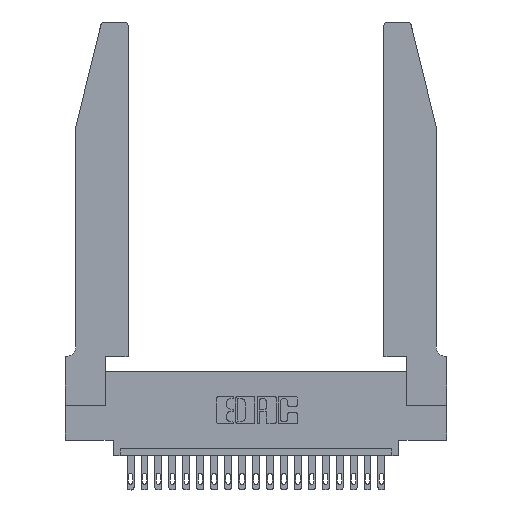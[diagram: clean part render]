
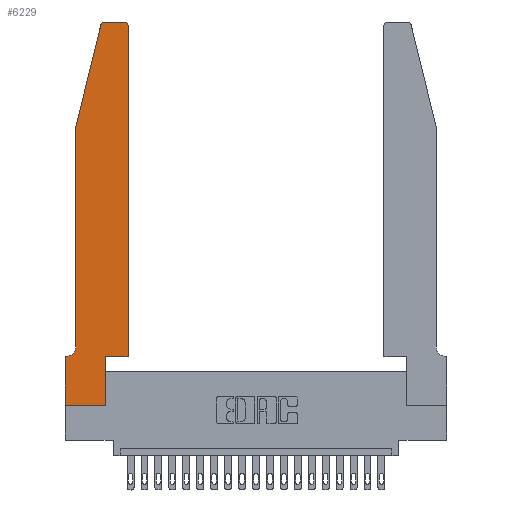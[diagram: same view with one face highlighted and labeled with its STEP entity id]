
A CAD part, top view. The second image highlights one B-rep face of the part: STEP entity #6229.
In plain terms, the highlighted planar face has unit normal (0, 0, 1).
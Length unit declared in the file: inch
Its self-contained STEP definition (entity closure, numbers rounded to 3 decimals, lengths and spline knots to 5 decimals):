
#37 = ORIENTED_EDGE ( 'NONE', *, *, #16105, .T. ) ;
#192 = DIRECTION ( 'NONE',  ( -1., 0., 0. ) ) ;
#451 = DIRECTION ( 'NONE',  ( 0., -1., 0. ) ) ;
#496 = ORIENTED_EDGE ( 'NONE', *, *, #21520, .T. ) ;
#1401 = AXIS2_PLACEMENT_3D ( 'NONE', #6919, #9205, #12466 ) ;
#1542 = VERTEX_POINT ( 'NONE', #12046 ) ;
#1591 = CIRCLE ( 'NONE', #13494, 0.03 ) ;
#1821 = DIRECTION ( 'NONE',  ( 0., -1., 0. ) ) ;
#2280 = EDGE_CURVE ( 'NONE', #3450, #8870, #7449, .T. ) ;
#2581 = VECTOR ( 'NONE', #192, 39.37008 ) ;
#2589 = VERTEX_POINT ( 'NONE', #8952 ) ;
#2864 = LINE ( 'NONE', #8711, #13382 ) ;
#3450 = VERTEX_POINT ( 'NONE', #17143 ) ;
#3491 = CARTESIAN_POINT ( 'NONE',  ( 0.2605, 2.75, 0.37 ) ) ;
#3514 = VERTEX_POINT ( 'NONE', #5051 ) ;
#3794 = PLANE ( 'NONE',  #1401 ) ;
#3999 = CARTESIAN_POINT ( 'NONE',  ( 0.0755, 2., 0.37 ) ) ;
#4789 = EDGE_CURVE ( 'NONE', #6012, #9250, #21505, .T. ) ;
#5051 = CARTESIAN_POINT ( 'NONE',  ( 0., 0., 0.37 ) ) ;
#5830 = DIRECTION ( 'NONE',  ( -0.239, -0.971, 0. ) ) ;
#6012 = VERTEX_POINT ( 'NONE', #11234 ) ;
#6162 = CIRCLE ( 'NONE', #18378, 0.03 ) ;
#6229 = ADVANCED_FACE ( 'NONE', ( #20666 ), #3794, .T. ) ;
#6919 = CARTESIAN_POINT ( 'NONE',  ( 0., 0.35, 0.37 ) ) ;
#7022 = VECTOR ( 'NONE', #11692, 39.37008 ) ;
#7136 = ORIENTED_EDGE ( 'NONE', *, *, #7549, .T. ) ;
#7192 = LINE ( 'NONE', #3999, #13911 ) ;
#7449 = LINE ( 'NONE', #3491, #2581 ) ;
#7549 = EDGE_CURVE ( 'NONE', #8870, #2589, #6162, .T. ) ;
#8025 = CARTESIAN_POINT ( 'NONE',  ( 0.0755, 0.42, 0.37 ) ) ;
#8158 = DIRECTION ( 'NONE',  ( 1., 0., 0. ) ) ;
#8570 = LINE ( 'NONE', #20771, #21968 ) ;
#8609 = VECTOR ( 'NONE', #17797, 39.37008 ) ;
#8654 = CARTESIAN_POINT ( 'NONE',  ( 0.0755, 2., 0.37 ) ) ;
#8711 = CARTESIAN_POINT ( 'NONE',  ( 0.0755, 0.35, 0.37 ) ) ;
#8735 = VERTEX_POINT ( 'NONE', #8025 ) ;
#8870 = VERTEX_POINT ( 'NONE', #16447 ) ;
#8952 = CARTESIAN_POINT ( 'NONE',  ( 0.25487, 2.72718, 0.37 ) ) ;
#9149 = LINE ( 'NONE', #13508, #7022 ) ;
#9182 = LINE ( 'NONE', #10750, #19371 ) ;
#9205 = DIRECTION ( 'NONE',  ( 0., 0., 1. ) ) ;
#9250 = VERTEX_POINT ( 'NONE', #13662 ) ;
#9502 = CARTESIAN_POINT ( 'NONE',  ( 0.0055, 0.35, 0.37 ) ) ;
#9859 = DIRECTION ( 'NONE',  ( 0., 0., -1. ) ) ;
#9960 = EDGE_CURVE ( 'NONE', #8735, #15627, #15907, .T. ) ;
#10392 = CARTESIAN_POINT ( 'NONE',  ( 0.284, 2.72, 0.37 ) ) ;
#10475 = EDGE_LOOP ( 'NONE', ( #19475, #7136, #37, #14950, #15733, #496, #14463, #22172, #17162, #10963, #10596, #19961 ) ) ;
#10504 = VECTOR ( 'NONE', #12929, 39.37008 ) ;
#10596 = ORIENTED_EDGE ( 'NONE', *, *, #11024, .T. ) ;
#10750 = CARTESIAN_POINT ( 'NONE',  ( 0.0755, 2., 0.37 ) ) ;
#10822 = CARTESIAN_POINT ( 'NONE',  ( 0.2865, 0.35, 0.37 ) ) ;
#10891 = CARTESIAN_POINT ( 'NONE',  ( 0.4505, 0.35, 0.37 ) ) ;
#10892 = DIRECTION ( 'NONE',  ( 0., 1., 0. ) ) ;
#10963 = ORIENTED_EDGE ( 'NONE', *, *, #20581, .T. ) ;
#11024 = EDGE_CURVE ( 'NONE', #1542, #12797, #16920, .T. ) ;
#11234 = CARTESIAN_POINT ( 'NONE',  ( 0.2865, 0., 0.37 ) ) ;
#11542 = VERTEX_POINT ( 'NONE', #20821 ) ;
#11692 = DIRECTION ( 'NONE',  ( 1., 0., 0. ) ) ;
#11704 = EDGE_CURVE ( 'NONE', #12797, #3450, #1591, .T. ) ;
#12046 = CARTESIAN_POINT ( 'NONE',  ( 0.4505, 0.35, 0.37 ) ) ;
#12466 = DIRECTION ( 'NONE',  ( 1., 0., 0. ) ) ;
#12501 = EDGE_CURVE ( 'NONE', #11542, #3514, #8570, .T. ) ;
#12797 = VERTEX_POINT ( 'NONE', #21436 ) ;
#12816 = CARTESIAN_POINT ( 'NONE',  ( 0.0055, 0.42, 0.37 ) ) ;
#12929 = DIRECTION ( 'NONE',  ( 1., 0., 0. ) ) ;
#12979 = VECTOR ( 'NONE', #10892, 39.37008 ) ;
#13145 = DIRECTION ( 'NONE',  ( 0., 0., 1. ) ) ;
#13382 = VECTOR ( 'NONE', #20678, 39.37008 ) ;
#13494 = AXIS2_PLACEMENT_3D ( 'NONE', #14638, #13145, #8158 ) ;
#13508 = CARTESIAN_POINT ( 'NONE',  ( 0.4505, 0.35, 0.37 ) ) ;
#13662 = CARTESIAN_POINT ( 'NONE',  ( 0.2865, 0.35, 0.37 ) ) ;
#13723 = DIRECTION ( 'NONE',  ( 1., 0., 0. ) ) ;
#13911 = VECTOR ( 'NONE', #5830, 39.37008 ) ;
#14271 = LINE ( 'NONE', #19547, #10504 ) ;
#14463 = ORIENTED_EDGE ( 'NONE', *, *, #12501, .T. ) ;
#14638 = CARTESIAN_POINT ( 'NONE',  ( 0.4205, 2.72, 0.37 ) ) ;
#14950 = ORIENTED_EDGE ( 'NONE', *, *, #19392, .T. ) ;
#15017 = DIRECTION ( 'NONE',  ( -1., 0., 0. ) ) ;
#15627 = VERTEX_POINT ( 'NONE', #9502 ) ;
#15733 = ORIENTED_EDGE ( 'NONE', *, *, #9960, .T. ) ;
#15907 = CIRCLE ( 'NONE', #19266, 0.07 ) ;
#16105 = EDGE_CURVE ( 'NONE', #2589, #16556, #7192, .T. ) ;
#16447 = CARTESIAN_POINT ( 'NONE',  ( 0.284, 2.75, 0.37 ) ) ;
#16556 = VERTEX_POINT ( 'NONE', #8654 ) ;
#16920 = LINE ( 'NONE', #10891, #8609 ) ;
#17070 = DIRECTION ( 'NONE',  ( 0., 0., 1. ) ) ;
#17143 = CARTESIAN_POINT ( 'NONE',  ( 0.4205, 2.75, 0.37 ) ) ;
#17162 = ORIENTED_EDGE ( 'NONE', *, *, #4789, .T. ) ;
#17797 = DIRECTION ( 'NONE',  ( 0., 1., 0. ) ) ;
#18378 = AXIS2_PLACEMENT_3D ( 'NONE', #10392, #17070, #13723 ) ;
#19266 = AXIS2_PLACEMENT_3D ( 'NONE', #12816, #9859, #15017 ) ;
#19371 = VECTOR ( 'NONE', #451, 39.37008 ) ;
#19392 = EDGE_CURVE ( 'NONE', #16556, #8735, #9182, .T. ) ;
#19475 = ORIENTED_EDGE ( 'NONE', *, *, #2280, .T. ) ;
#19547 = CARTESIAN_POINT ( 'NONE',  ( 0., 0., 0.37 ) ) ;
#19961 = ORIENTED_EDGE ( 'NONE', *, *, #11704, .T. ) ;
#20185 = EDGE_CURVE ( 'NONE', #3514, #6012, #14271, .T. ) ;
#20581 = EDGE_CURVE ( 'NONE', #9250, #1542, #9149, .T. ) ;
#20666 = FACE_OUTER_BOUND ( 'NONE', #10475, .T. ) ;
#20678 = DIRECTION ( 'NONE',  ( -1., 0., 0. ) ) ;
#20771 = CARTESIAN_POINT ( 'NONE',  ( 0., 0., 0.37 ) ) ;
#20821 = CARTESIAN_POINT ( 'NONE',  ( 0., 0.35, 0.37 ) ) ;
#21436 = CARTESIAN_POINT ( 'NONE',  ( 0.4505, 2.72, 0.37 ) ) ;
#21505 = LINE ( 'NONE', #10822, #12979 ) ;
#21520 = EDGE_CURVE ( 'NONE', #15627, #11542, #2864, .T. ) ;
#21968 = VECTOR ( 'NONE', #1821, 39.37008 ) ;
#22172 = ORIENTED_EDGE ( 'NONE', *, *, #20185, .T. ) ;
